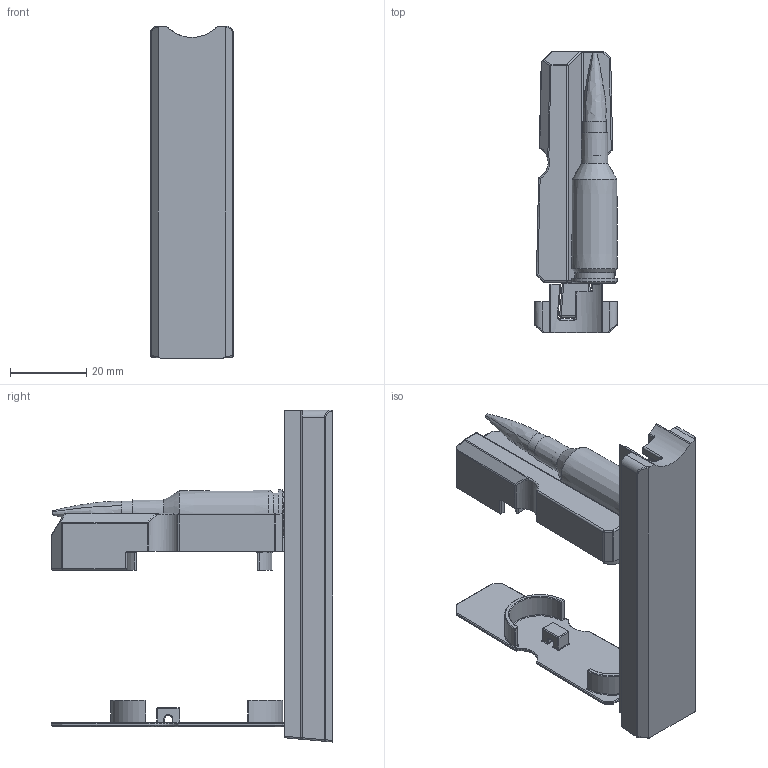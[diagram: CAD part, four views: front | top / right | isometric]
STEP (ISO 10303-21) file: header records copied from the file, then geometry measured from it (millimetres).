
FILE_DESCRIPTION(/* description */ (''),/* implementation_level */ '2;1');
FILE_NAME(/* name */ 'aw_magazine_6br_kit.step',/* time_stamp */ '2024-03-10T22:08:27+13:00',/* author */ (''),/* organization */ (''),/* preprocessor_version */ 'ST-DEVELOPER v20',/* originating_system */ 'Autodesk Translation Framework v12.20.1.177',/* authorisation */ '');
FILE_SCHEMA (('AUTOMOTIVE_DESIGN { 1 0 10303 214 3 1 1 }'));
Length unit declared in the file: millimetre
Products named in the file (4): aw_magazine_6br_kit; 6mmbr_dummy_round; 6mmbr brass; berger_109gr_long_range_hybrid
Assembly tree (3 placements, depth 3):
  aw_magazine_6br_kit
    6mmbr_dummy_round
      6mmbr brass
      berger_109gr_long_range_hybrid
Bounding box: 21.77 x 73.8 x 87 mm (x, y, z)
Volume: 29179.1 mm3; surface area: 17374.4 mm2
Topology: 5 solids, 5 shells, 723 faces, 1807 edges, 1094 vertices
Faces by surface type: plane 292, bspline 172, cylinder 140, cone 66, torus 32, sphere 21
Full cylindrical faces by diameter (mm): 4.45 x1, 6.172 x1, 10.39 x1, 12.01 x1
Entity records: 26823 total; most frequent: CARTESIAN_POINT 10580, ORIENTED_EDGE 3554, DIRECTION 2963, EDGE_CURVE 1777, VERTEX_POINT 1094, LINE 1061, VECTOR 1061, AXIS2_PLACEMENT_3D 951
